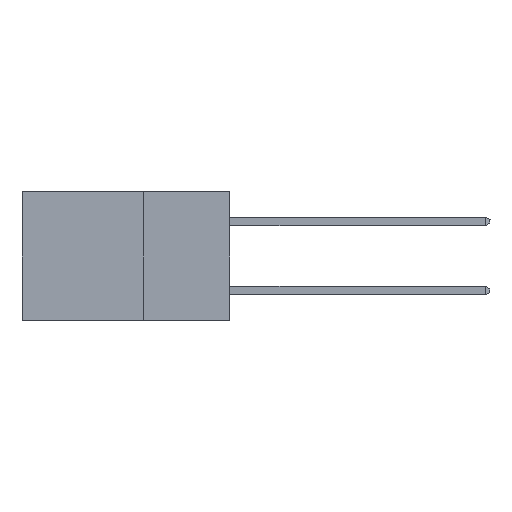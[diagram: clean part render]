
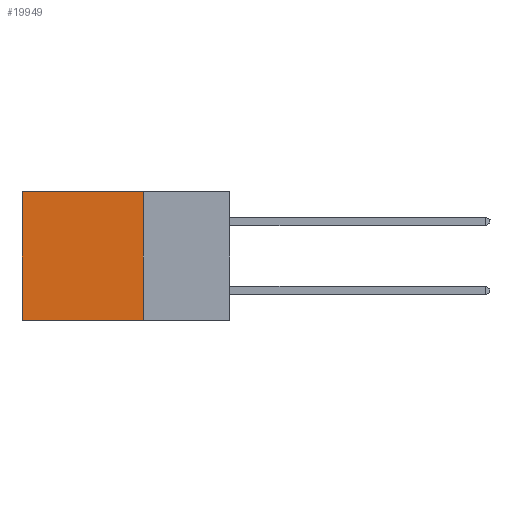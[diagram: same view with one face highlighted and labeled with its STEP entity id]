
A CAD part, left-side view. The second image highlights one B-rep face of the part: STEP entity #19949.
In plain terms, the highlighted planar face has unit normal (-1, 0, 0).
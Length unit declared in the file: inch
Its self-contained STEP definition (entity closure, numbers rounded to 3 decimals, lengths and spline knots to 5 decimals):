
#803 = LINE ( 'NONE', #4372, #18386 ) ;
#1908 = VECTOR ( 'NONE', #14525, 39.37008 ) ;
#2492 = VERTEX_POINT ( 'NONE', #11393 ) ;
#2837 = DIRECTION ( 'NONE',  ( 0., 0., -1. ) ) ;
#2904 = ORIENTED_EDGE ( 'NONE', *, *, #3162, .F. ) ;
#3162 = EDGE_CURVE ( 'NONE', #9970, #21008, #803, .T. ) ;
#3697 = LINE ( 'NONE', #18485, #5485 ) ;
#4185 = CARTESIAN_POINT ( 'NONE',  ( 0.2615, 0.6, -0.37 ) ) ;
#4372 = CARTESIAN_POINT ( 'NONE',  ( 0.2615, 0.25, -0.37 ) ) ;
#4781 = CARTESIAN_POINT ( 'NONE',  ( 0.2615, 0.25, 0. ) ) ;
#4811 = FACE_OUTER_BOUND ( 'NONE', #6971, .T. ) ;
#5271 = CARTESIAN_POINT ( 'NONE',  ( 0.2615, 0.6, -0.37 ) ) ;
#5485 = VECTOR ( 'NONE', #5606, 39.37008 ) ;
#5606 = DIRECTION ( 'NONE',  ( 0., 1., 0. ) ) ;
#5713 = EDGE_CURVE ( 'NONE', #9970, #2492, #19359, .T. ) ;
#6102 = DIRECTION ( 'NONE',  ( 1., 0., 0. ) ) ;
#6971 = EDGE_LOOP ( 'NONE', ( #11362, #14354, #2904, #10007 ) ) ;
#7217 = VERTEX_POINT ( 'NONE', #4185 ) ;
#7907 = PLANE ( 'NONE',  #16574 ) ;
#8121 = CARTESIAN_POINT ( 'NONE',  ( 0.2615, 0.25, -0.37 ) ) ;
#9970 = VERTEX_POINT ( 'NONE', #13908 ) ;
#10007 = ORIENTED_EDGE ( 'NONE', *, *, #5713, .T. ) ;
#11142 = DIRECTION ( 'NONE',  ( 0., 0., -1. ) ) ;
#11362 = ORIENTED_EDGE ( 'NONE', *, *, #16884, .T. ) ;
#11393 = CARTESIAN_POINT ( 'NONE',  ( 0.2615, 0.6, 0. ) ) ;
#12031 = DIRECTION ( 'NONE',  ( 0., 0., -1. ) ) ;
#12255 = CARTESIAN_POINT ( 'NONE',  ( 0.2615, 0.25, -0.37 ) ) ;
#13908 = CARTESIAN_POINT ( 'NONE',  ( 0.2615, 0.25, 0. ) ) ;
#14354 = ORIENTED_EDGE ( 'NONE', *, *, #17774, .F. ) ;
#14525 = DIRECTION ( 'NONE',  ( 0., 1., 0. ) ) ;
#16574 = AXIS2_PLACEMENT_3D ( 'NONE', #8121, #6102, #11142 ) ;
#16760 = VECTOR ( 'NONE', #12031, 39.37008 ) ;
#16884 = EDGE_CURVE ( 'NONE', #2492, #7217, #19970, .T. ) ;
#17774 = EDGE_CURVE ( 'NONE', #21008, #7217, #3697, .T. ) ;
#18386 = VECTOR ( 'NONE', #2837, 39.37008 ) ;
#18485 = CARTESIAN_POINT ( 'NONE',  ( 0.2615, 0.25, -0.37 ) ) ;
#19359 = LINE ( 'NONE', #4781, #1908 ) ;
#19949 = ADVANCED_FACE ( 'NONE', ( #4811 ), #7907, .F. ) ;
#19970 = LINE ( 'NONE', #5271, #16760 ) ;
#21008 = VERTEX_POINT ( 'NONE', #12255 ) ;
